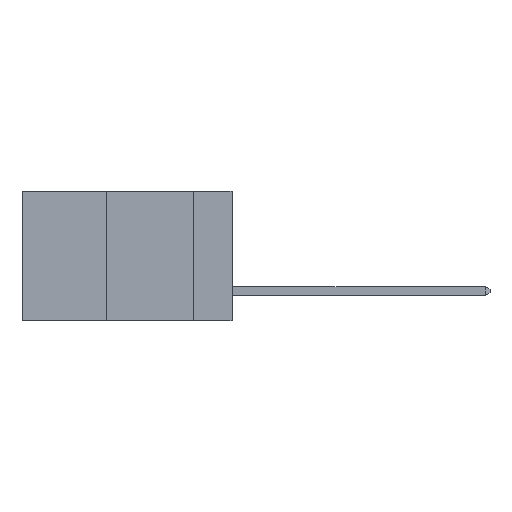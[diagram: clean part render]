
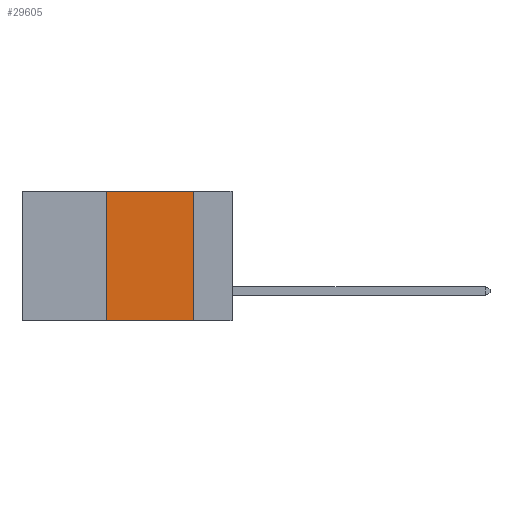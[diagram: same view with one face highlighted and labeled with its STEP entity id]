
A CAD part, left-side view. The second image highlights one B-rep face of the part: STEP entity #29605.
In plain terms, the highlighted planar face has unit normal (-1, 0, 0).
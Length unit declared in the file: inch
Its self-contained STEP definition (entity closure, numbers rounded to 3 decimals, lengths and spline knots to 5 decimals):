
#957 = DIRECTION ( 'NONE',  ( 0., 0., -1. ) ) ;
#1563 = CARTESIAN_POINT ( 'NONE',  ( 0., 0.36, -0.37 ) ) ;
#2787 = VECTOR ( 'NONE', #5510, 39.37008 ) ;
#3467 = VERTEX_POINT ( 'NONE', #18098 ) ;
#3652 = LINE ( 'NONE', #5631, #2787 ) ;
#3679 = CARTESIAN_POINT ( 'NONE',  ( 0., 0.11, -0.37 ) ) ;
#3888 = LINE ( 'NONE', #27146, #31140 ) ;
#4022 = AXIS2_PLACEMENT_3D ( 'NONE', #14731, #17459, #957 ) ;
#4603 = CARTESIAN_POINT ( 'NONE',  ( 0., 0.11, 0. ) ) ;
#4854 = VECTOR ( 'NONE', #14115, 39.37008 ) ;
#5363 = EDGE_CURVE ( 'NONE', #3467, #17599, #19390, .T. ) ;
#5510 = DIRECTION ( 'NONE',  ( 0., 0., 1. ) ) ;
#5631 = CARTESIAN_POINT ( 'NONE',  ( 0., 0.36, 0. ) ) ;
#10387 = VECTOR ( 'NONE', #26360, 39.37008 ) ;
#12386 = FACE_OUTER_BOUND ( 'NONE', #13531, .T. ) ;
#13531 = EDGE_LOOP ( 'NONE', ( #28407, #14062, #21990, #20424 ) ) ;
#14062 = ORIENTED_EDGE ( 'NONE', *, *, #5363, .F. ) ;
#14115 = DIRECTION ( 'NONE',  ( 0., -1., 0. ) ) ;
#14731 = CARTESIAN_POINT ( 'NONE',  ( 0., 0.6, 0. ) ) ;
#17459 = DIRECTION ( 'NONE',  ( 1., 0., 0. ) ) ;
#17599 = VERTEX_POINT ( 'NONE', #27834 ) ;
#18098 = CARTESIAN_POINT ( 'NONE',  ( 0., 0.36, 0. ) ) ;
#19052 = DIRECTION ( 'NONE',  ( 0., -1., 0. ) ) ;
#19390 = LINE ( 'NONE', #33001, #4854 ) ;
#20424 = ORIENTED_EDGE ( 'NONE', *, *, #31096, .T. ) ;
#20788 = VERTEX_POINT ( 'NONE', #3679 ) ;
#21990 = ORIENTED_EDGE ( 'NONE', *, *, #25391, .F. ) ;
#25391 = EDGE_CURVE ( 'NONE', #34779, #3467, #3652, .T. ) ;
#25629 = LINE ( 'NONE', #4603, #10387 ) ;
#26360 = DIRECTION ( 'NONE',  ( 0., 0., -1. ) ) ;
#27146 = CARTESIAN_POINT ( 'NONE',  ( 0., 0.6, -0.37 ) ) ;
#27834 = CARTESIAN_POINT ( 'NONE',  ( 0., 0.11, 0. ) ) ;
#28407 = ORIENTED_EDGE ( 'NONE', *, *, #34869, .F. ) ;
#29605 = ADVANCED_FACE ( 'NONE', ( #12386 ), #30907, .F. ) ;
#30907 = PLANE ( 'NONE',  #4022 ) ;
#31096 = EDGE_CURVE ( 'NONE', #34779, #20788, #3888, .T. ) ;
#31140 = VECTOR ( 'NONE', #19052, 39.37008 ) ;
#33001 = CARTESIAN_POINT ( 'NONE',  ( 0., 0.6, 0. ) ) ;
#34779 = VERTEX_POINT ( 'NONE', #1563 ) ;
#34869 = EDGE_CURVE ( 'NONE', #17599, #20788, #25629, .T. ) ;
